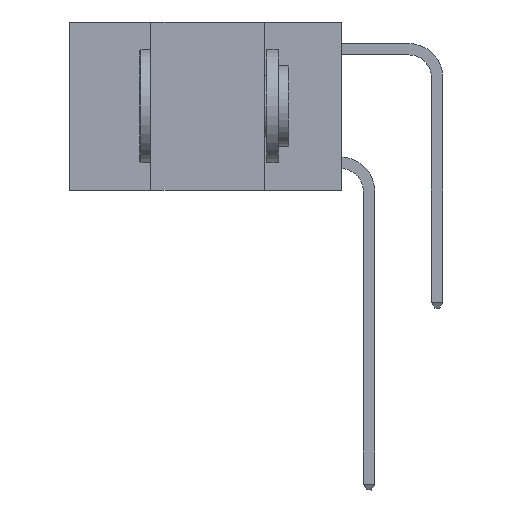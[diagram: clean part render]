
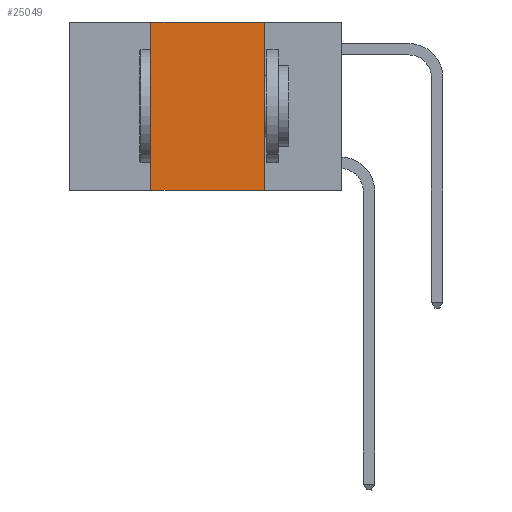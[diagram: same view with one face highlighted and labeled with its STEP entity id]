
A CAD part, left-side view. The second image highlights one B-rep face of the part: STEP entity #25049.
In plain terms, the highlighted planar face has unit normal (-1, 0, 0).
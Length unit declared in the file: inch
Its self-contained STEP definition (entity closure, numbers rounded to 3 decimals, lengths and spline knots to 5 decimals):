
#858 = DIRECTION ( 'NONE',  ( 0., 0., -1. ) ) ;
#1371 = AXIS2_PLACEMENT_3D ( 'NONE', #15398, #12659, #30894 ) ;
#2221 = DIRECTION ( 'NONE',  ( 0., -1., 0. ) ) ;
#2462 = VERTEX_POINT ( 'NONE', #18143 ) ;
#2621 = PLANE ( 'NONE',  #1371 ) ;
#2860 = LINE ( 'NONE', #12736, #25281 ) ;
#3919 = EDGE_LOOP ( 'NONE', ( #10768, #19222, #4454, #12305 ) ) ;
#4421 = VERTEX_POINT ( 'NONE', #21170 ) ;
#4454 = ORIENTED_EDGE ( 'NONE', *, *, #12836, .F. ) ;
#5241 = EDGE_CURVE ( 'NONE', #4421, #18968, #16477, .T. ) ;
#10768 = ORIENTED_EDGE ( 'NONE', *, *, #16495, .F. ) ;
#12132 = CARTESIAN_POINT ( 'NONE',  ( 0., 0.42, 0. ) ) ;
#12305 = ORIENTED_EDGE ( 'NONE', *, *, #14582, .T. ) ;
#12659 = DIRECTION ( 'NONE',  ( 1., 0., 0. ) ) ;
#12736 = CARTESIAN_POINT ( 'NONE',  ( 0., 0.6, -0.37 ) ) ;
#12794 = VECTOR ( 'NONE', #22494, 39.37008 ) ;
#12836 = EDGE_CURVE ( 'NONE', #19937, #4421, #27193, .T. ) ;
#13174 = CARTESIAN_POINT ( 'NONE',  ( 0., 0.17, 0. ) ) ;
#13375 = VECTOR ( 'NONE', #858, 39.37008 ) ;
#14411 = CARTESIAN_POINT ( 'NONE',  ( 0., 0.17, 0. ) ) ;
#14582 = EDGE_CURVE ( 'NONE', #19937, #2462, #2860, .T. ) ;
#15398 = CARTESIAN_POINT ( 'NONE',  ( 0., 0.6, 0. ) ) ;
#16477 = LINE ( 'NONE', #16805, #21081 ) ;
#16495 = EDGE_CURVE ( 'NONE', #18968, #2462, #25495, .T. ) ;
#16805 = CARTESIAN_POINT ( 'NONE',  ( 0., 0.6, 0. ) ) ;
#18143 = CARTESIAN_POINT ( 'NONE',  ( 0., 0.17, -0.37 ) ) ;
#18968 = VERTEX_POINT ( 'NONE', #14411 ) ;
#19222 = ORIENTED_EDGE ( 'NONE', *, *, #5241, .F. ) ;
#19937 = VERTEX_POINT ( 'NONE', #29217 ) ;
#21081 = VECTOR ( 'NONE', #2221, 39.37008 ) ;
#21170 = CARTESIAN_POINT ( 'NONE',  ( 0., 0.42, 0. ) ) ;
#22494 = DIRECTION ( 'NONE',  ( 0., 0., 1. ) ) ;
#22632 = DIRECTION ( 'NONE',  ( 0., -1., 0. ) ) ;
#24974 = FACE_OUTER_BOUND ( 'NONE', #3919, .T. ) ;
#25049 = ADVANCED_FACE ( 'NONE', ( #24974 ), #2621, .F. ) ;
#25281 = VECTOR ( 'NONE', #22632, 39.37008 ) ;
#25495 = LINE ( 'NONE', #13174, #13375 ) ;
#27193 = LINE ( 'NONE', #12132, #12794 ) ;
#29217 = CARTESIAN_POINT ( 'NONE',  ( 0., 0.42, -0.37 ) ) ;
#30894 = DIRECTION ( 'NONE',  ( 0., 0., -1. ) ) ;
